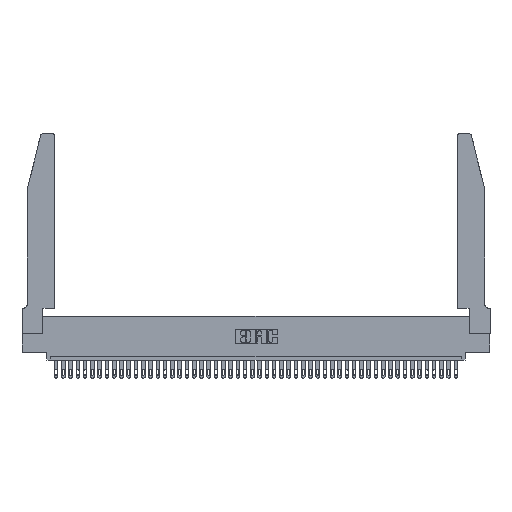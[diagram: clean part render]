
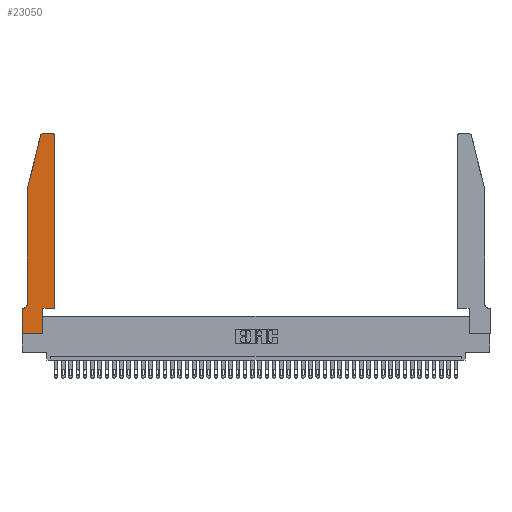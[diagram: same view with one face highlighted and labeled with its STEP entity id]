
A CAD part, top view. The second image highlights one B-rep face of the part: STEP entity #23050.
In plain terms, the highlighted planar face has unit normal (0, 0, 1).
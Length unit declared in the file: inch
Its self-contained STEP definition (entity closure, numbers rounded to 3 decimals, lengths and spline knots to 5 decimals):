
#62 = LINE ( 'NONE', #12165, #15786 ) ;
#633 = EDGE_CURVE ( 'NONE', #35044, #34530, #9407, .T. ) ;
#1574 = ORIENTED_EDGE ( 'NONE', *, *, #36677, .T. ) ;
#1776 = AXIS2_PLACEMENT_3D ( 'NONE', #27634, #10266, #41775 ) ;
#2123 = DIRECTION ( 'NONE',  ( 0., 0., -1. ) ) ;
#2533 = VECTOR ( 'NONE', #8104, 39.37008 ) ;
#3511 = VERTEX_POINT ( 'NONE', #4433 ) ;
#3661 = AXIS2_PLACEMENT_3D ( 'NONE', #42277, #38554, #3880 ) ;
#3880 = DIRECTION ( 'NONE',  ( 1., 0., 0. ) ) ;
#4122 = DIRECTION ( 'NONE',  ( 1., 0., 0. ) ) ;
#4199 = CARTESIAN_POINT ( 'NONE',  ( 0.0755, 0.42, 0.37 ) ) ;
#4433 = CARTESIAN_POINT ( 'NONE',  ( 0.0055, 0.35, 0.37 ) ) ;
#4753 = EDGE_CURVE ( 'NONE', #24633, #23197, #13344, .T. ) ;
#5020 = LINE ( 'NONE', #31054, #20788 ) ;
#5870 = CARTESIAN_POINT ( 'NONE',  ( 0.2865, 0., 0.37 ) ) ;
#7728 = CARTESIAN_POINT ( 'NONE',  ( 0.4505, 0.35, 0.37 ) ) ;
#8104 = DIRECTION ( 'NONE',  ( 0., 1., 0. ) ) ;
#8507 = ORIENTED_EDGE ( 'NONE', *, *, #38413, .T. ) ;
#8567 = ORIENTED_EDGE ( 'NONE', *, *, #27597, .T. ) ;
#8777 = EDGE_CURVE ( 'NONE', #37673, #24956, #9702, .T. ) ;
#8892 = DIRECTION ( 'NONE',  ( -1., 0., 0. ) ) ;
#9407 = CIRCLE ( 'NONE', #3661, 0.03 ) ;
#9702 = LINE ( 'NONE', #13663, #19970 ) ;
#10266 = DIRECTION ( 'NONE',  ( 0., 0., 1. ) ) ;
#11715 = VECTOR ( 'NONE', #33940, 39.37008 ) ;
#12165 = CARTESIAN_POINT ( 'NONE',  ( 0.0755, 0.35, 0.37 ) ) ;
#12783 = DIRECTION ( 'NONE',  ( -1., 0., 0. ) ) ;
#13344 = LINE ( 'NONE', #16791, #26945 ) ;
#13663 = CARTESIAN_POINT ( 'NONE',  ( 0., 0., 0.37 ) ) ;
#13852 = VERTEX_POINT ( 'NONE', #43696 ) ;
#14514 = VERTEX_POINT ( 'NONE', #27146 ) ;
#14810 = VERTEX_POINT ( 'NONE', #28896 ) ;
#15339 = CARTESIAN_POINT ( 'NONE',  ( 0.0755, 2., 0.37 ) ) ;
#15786 = VECTOR ( 'NONE', #12783, 39.37008 ) ;
#16554 = ORIENTED_EDGE ( 'NONE', *, *, #35403, .T. ) ;
#16791 = CARTESIAN_POINT ( 'NONE',  ( 0.0755, 2., 0.37 ) ) ;
#17064 = CARTESIAN_POINT ( 'NONE',  ( 0.284, 2.75, 0.37 ) ) ;
#18180 = EDGE_CURVE ( 'NONE', #3511, #37673, #62, .T. ) ;
#18228 = ORIENTED_EDGE ( 'NONE', *, *, #38913, .T. ) ;
#18911 = LINE ( 'NONE', #25428, #38637 ) ;
#19970 = VECTOR ( 'NONE', #44544, 39.37008 ) ;
#20318 = DIRECTION ( 'NONE',  ( 0., 0., 1. ) ) ;
#20726 = ORIENTED_EDGE ( 'NONE', *, *, #4753, .T. ) ;
#20788 = VECTOR ( 'NONE', #30433, 39.37008 ) ;
#21313 = ORIENTED_EDGE ( 'NONE', *, *, #633, .T. ) ;
#22956 = CARTESIAN_POINT ( 'NONE',  ( 0.0055, 0.42, 0.37 ) ) ;
#23050 = ADVANCED_FACE ( 'NONE', ( #34391 ), #44933, .T. ) ;
#23053 = ORIENTED_EDGE ( 'NONE', *, *, #40956, .T. ) ;
#23149 = ORIENTED_EDGE ( 'NONE', *, *, #18180, .T. ) ;
#23197 = VERTEX_POINT ( 'NONE', #4199 ) ;
#23390 = CIRCLE ( 'NONE', #34451, 0.07 ) ;
#23503 = CARTESIAN_POINT ( 'NONE',  ( 0.4205, 2.72, 0.37 ) ) ;
#24633 = VERTEX_POINT ( 'NONE', #15339 ) ;
#24749 = CARTESIAN_POINT ( 'NONE',  ( 0.0755, 2., 0.37 ) ) ;
#24956 = VERTEX_POINT ( 'NONE', #28756 ) ;
#25428 = CARTESIAN_POINT ( 'NONE',  ( 0., 0., 0.37 ) ) ;
#25818 = CIRCLE ( 'NONE', #42274, 0.03 ) ;
#26945 = VECTOR ( 'NONE', #34702, 39.37008 ) ;
#27146 = CARTESIAN_POINT ( 'NONE',  ( 0.2865, 0.35, 0.37 ) ) ;
#27162 = CARTESIAN_POINT ( 'NONE',  ( 0.2605, 2.75, 0.37 ) ) ;
#27597 = EDGE_CURVE ( 'NONE', #27700, #13852, #25818, .T. ) ;
#27634 = CARTESIAN_POINT ( 'NONE',  ( 0., 0.35, 0.37 ) ) ;
#27700 = VERTEX_POINT ( 'NONE', #35513 ) ;
#28316 = DIRECTION ( 'NONE',  ( -0.239, -0.971, 0. ) ) ;
#28738 = DIRECTION ( 'NONE',  ( 1., 0., 0. ) ) ;
#28756 = CARTESIAN_POINT ( 'NONE',  ( 0., 0., 0.37 ) ) ;
#28896 = CARTESIAN_POINT ( 'NONE',  ( 0.4505, 0.35, 0.37 ) ) ;
#28963 = CARTESIAN_POINT ( 'NONE',  ( 0.4505, 0.35, 0.37 ) ) ;
#30433 = DIRECTION ( 'NONE',  ( 0., 1., 0. ) ) ;
#31054 = CARTESIAN_POINT ( 'NONE',  ( 0.2865, 0.35, 0.37 ) ) ;
#31451 = CARTESIAN_POINT ( 'NONE',  ( 0.25487, 2.72718, 0.37 ) ) ;
#31990 = ORIENTED_EDGE ( 'NONE', *, *, #33474, .T. ) ;
#32112 = CARTESIAN_POINT ( 'NONE',  ( 0., 0.35, 0.37 ) ) ;
#32358 = ORIENTED_EDGE ( 'NONE', *, *, #44556, .T. ) ;
#32364 = DIRECTION ( 'NONE',  ( 1., 0., 0. ) ) ;
#33474 = EDGE_CURVE ( 'NONE', #13852, #35044, #42250, .T. ) ;
#33940 = DIRECTION ( 'NONE',  ( -1., 0., 0. ) ) ;
#34391 = FACE_OUTER_BOUND ( 'NONE', #39958, .T. ) ;
#34451 = AXIS2_PLACEMENT_3D ( 'NONE', #22956, #2123, #8892 ) ;
#34530 = VERTEX_POINT ( 'NONE', #31451 ) ;
#34702 = DIRECTION ( 'NONE',  ( 0., -1., 0. ) ) ;
#35044 = VERTEX_POINT ( 'NONE', #17064 ) ;
#35403 = EDGE_CURVE ( 'NONE', #39172, #14514, #5020, .T. ) ;
#35513 = CARTESIAN_POINT ( 'NONE',  ( 0.4505, 2.72, 0.37 ) ) ;
#36350 = LINE ( 'NONE', #28963, #2533 ) ;
#36677 = EDGE_CURVE ( 'NONE', #23197, #3511, #23390, .T. ) ;
#37673 = VERTEX_POINT ( 'NONE', #32112 ) ;
#38331 = VECTOR ( 'NONE', #28738, 39.37008 ) ;
#38413 = EDGE_CURVE ( 'NONE', #14810, #27700, #36350, .T. ) ;
#38554 = DIRECTION ( 'NONE',  ( 0., 0., 1. ) ) ;
#38637 = VECTOR ( 'NONE', #32364, 39.37008 ) ;
#38913 = EDGE_CURVE ( 'NONE', #34530, #24633, #40182, .T. ) ;
#39057 = VECTOR ( 'NONE', #28316, 39.37008 ) ;
#39172 = VERTEX_POINT ( 'NONE', #5870 ) ;
#39264 = ORIENTED_EDGE ( 'NONE', *, *, #8777, .T. ) ;
#39958 = EDGE_LOOP ( 'NONE', ( #31990, #21313, #18228, #20726, #1574, #23149, #39264, #32358, #16554, #23053, #8507, #8567 ) ) ;
#40182 = LINE ( 'NONE', #24749, #39057 ) ;
#40956 = EDGE_CURVE ( 'NONE', #14514, #14810, #41032, .T. ) ;
#41032 = LINE ( 'NONE', #7728, #38331 ) ;
#41775 = DIRECTION ( 'NONE',  ( 1., 0., 0. ) ) ;
#42250 = LINE ( 'NONE', #27162, #11715 ) ;
#42274 = AXIS2_PLACEMENT_3D ( 'NONE', #23503, #20318, #4122 ) ;
#42277 = CARTESIAN_POINT ( 'NONE',  ( 0.284, 2.72, 0.37 ) ) ;
#43696 = CARTESIAN_POINT ( 'NONE',  ( 0.4205, 2.75, 0.37 ) ) ;
#44544 = DIRECTION ( 'NONE',  ( 0., -1., 0. ) ) ;
#44556 = EDGE_CURVE ( 'NONE', #24956, #39172, #18911, .T. ) ;
#44933 = PLANE ( 'NONE',  #1776 ) ;
